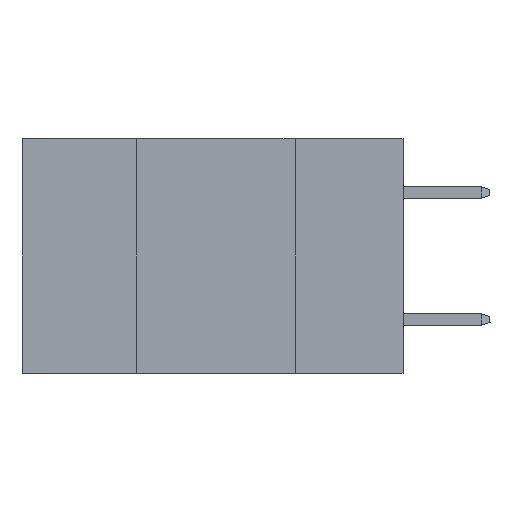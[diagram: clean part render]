
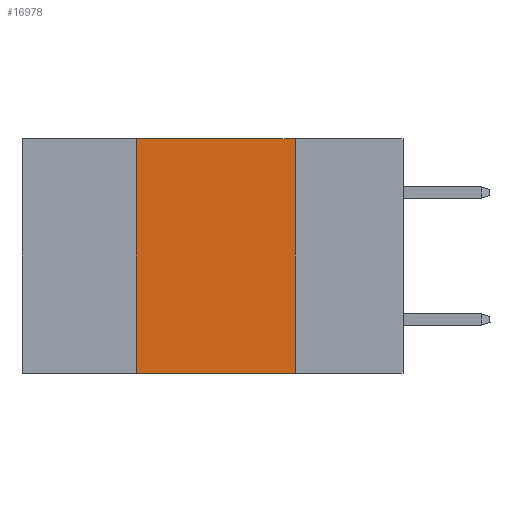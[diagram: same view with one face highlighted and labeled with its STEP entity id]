
A CAD part, left-side view. The second image highlights one B-rep face of the part: STEP entity #16978.
In plain terms, the highlighted planar face has unit normal (-1, 0, 0).
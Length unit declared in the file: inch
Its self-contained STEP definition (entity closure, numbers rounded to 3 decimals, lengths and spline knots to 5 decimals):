
#161 = VECTOR ( 'NONE', #13655, 39.37008 ) ;
#185 = EDGE_CURVE ( 'NONE', #17704, #16861, #17194, .T. ) ;
#1688 = LINE ( 'NONE', #22951, #22025 ) ;
#1841 = DIRECTION ( 'NONE',  ( 1., 0., 0. ) ) ;
#2051 = VECTOR ( 'NONE', #15947, 39.37008 ) ;
#3861 = EDGE_CURVE ( 'NONE', #21239, #17704, #1688, .T. ) ;
#3920 = CARTESIAN_POINT ( 'NONE',  ( 0., 0.42, 0. ) ) ;
#5195 = EDGE_CURVE ( 'NONE', #7220, #21239, #21151, .T. ) ;
#5199 = ORIENTED_EDGE ( 'NONE', *, *, #5195, .F. ) ;
#5495 = LINE ( 'NONE', #21668, #15845 ) ;
#5718 = DIRECTION ( 'NONE',  ( 0., -1., 0. ) ) ;
#5745 = DIRECTION ( 'NONE',  ( 0., 0., -1. ) ) ;
#7220 = VERTEX_POINT ( 'NONE', #22052 ) ;
#8371 = CARTESIAN_POINT ( 'NONE',  ( 0., 0.17, 0. ) ) ;
#8918 = EDGE_LOOP ( 'NONE', ( #15106, #13456, #5199, #18060 ) ) ;
#9516 = AXIS2_PLACEMENT_3D ( 'NONE', #21693, #1841, #5745 ) ;
#10380 = CARTESIAN_POINT ( 'NONE',  ( 0., 0.17, -0.37 ) ) ;
#12639 = EDGE_CURVE ( 'NONE', #7220, #16861, #5495, .T. ) ;
#13456 = ORIENTED_EDGE ( 'NONE', *, *, #3861, .F. ) ;
#13655 = DIRECTION ( 'NONE',  ( 0., 0., -1. ) ) ;
#15106 = ORIENTED_EDGE ( 'NONE', *, *, #185, .F. ) ;
#15845 = VECTOR ( 'NONE', #5718, 39.37008 ) ;
#15947 = DIRECTION ( 'NONE',  ( 0., 0., 1. ) ) ;
#16386 = FACE_OUTER_BOUND ( 'NONE', #8918, .T. ) ;
#16861 = VERTEX_POINT ( 'NONE', #10380 ) ;
#16978 = ADVANCED_FACE ( 'NONE', ( #16386 ), #21929, .F. ) ;
#17194 = LINE ( 'NONE', #20850, #161 ) ;
#17704 = VERTEX_POINT ( 'NONE', #8371 ) ;
#18060 = ORIENTED_EDGE ( 'NONE', *, *, #12639, .T. ) ;
#19435 = DIRECTION ( 'NONE',  ( 0., -1., 0. ) ) ;
#19436 = CARTESIAN_POINT ( 'NONE',  ( 0., 0.42, 0. ) ) ;
#20850 = CARTESIAN_POINT ( 'NONE',  ( 0., 0.17, 0. ) ) ;
#21151 = LINE ( 'NONE', #3920, #2051 ) ;
#21239 = VERTEX_POINT ( 'NONE', #19436 ) ;
#21668 = CARTESIAN_POINT ( 'NONE',  ( 0., 0.6, -0.37 ) ) ;
#21693 = CARTESIAN_POINT ( 'NONE',  ( 0., 0.6, 0. ) ) ;
#21929 = PLANE ( 'NONE',  #9516 ) ;
#22025 = VECTOR ( 'NONE', #19435, 39.37008 ) ;
#22052 = CARTESIAN_POINT ( 'NONE',  ( 0., 0.42, -0.37 ) ) ;
#22951 = CARTESIAN_POINT ( 'NONE',  ( 0., 0.6, 0. ) ) ;
